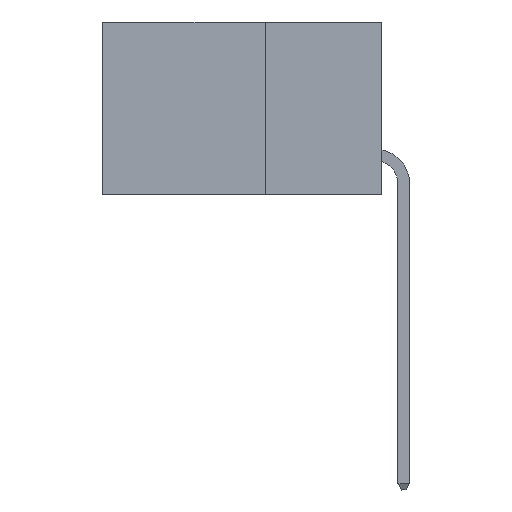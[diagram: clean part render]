
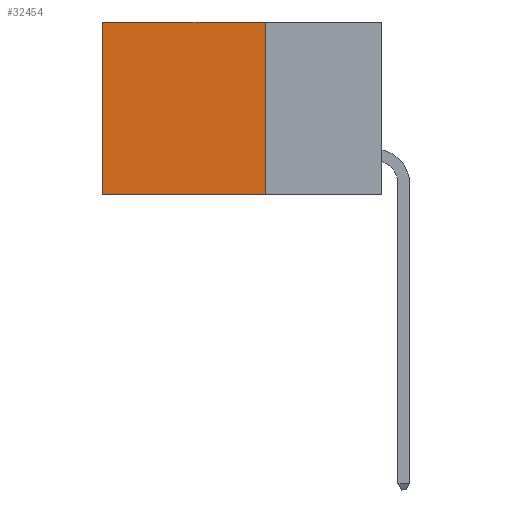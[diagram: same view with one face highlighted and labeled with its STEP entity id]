
A CAD part, left-side view. The second image highlights one B-rep face of the part: STEP entity #32454.
In plain terms, the highlighted planar face has unit normal (-1, 0, 0).
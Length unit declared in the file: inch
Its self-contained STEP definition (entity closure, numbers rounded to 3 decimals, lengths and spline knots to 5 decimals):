
#562 = CARTESIAN_POINT ( 'NONE',  ( 0.2875, 0.25, -0.37 ) ) ;
#2887 = CARTESIAN_POINT ( 'NONE',  ( 0.2875, 0.25, 0. ) ) ;
#3276 = LINE ( 'NONE', #2887, #10043 ) ;
#3632 = VECTOR ( 'NONE', #9396, 39.37008 ) ;
#3979 = CARTESIAN_POINT ( 'NONE',  ( 0.2875, 0.25, 0. ) ) ;
#5584 = VERTEX_POINT ( 'NONE', #30612 ) ;
#6220 = ORIENTED_EDGE ( 'NONE', *, *, #30101, .T. ) ;
#6611 = EDGE_LOOP ( 'NONE', ( #34724, #22418, #9302, #6220 ) ) ;
#6703 = DIRECTION ( 'NONE',  ( 1., 0., 0. ) ) ;
#8087 = DIRECTION ( 'NONE',  ( 0., 1., 0. ) ) ;
#8791 = VECTOR ( 'NONE', #34684, 39.37008 ) ;
#9302 = ORIENTED_EDGE ( 'NONE', *, *, #34766, .F. ) ;
#9396 = DIRECTION ( 'NONE',  ( 0., 0., -1. ) ) ;
#10043 = VECTOR ( 'NONE', #16266, 39.37008 ) ;
#10586 = FACE_OUTER_BOUND ( 'NONE', #6611, .T. ) ;
#15884 = CARTESIAN_POINT ( 'NONE',  ( 0.2875, 0.25, 0. ) ) ;
#15912 = LINE ( 'NONE', #15884, #8791 ) ;
#16266 = DIRECTION ( 'NONE',  ( 0., 0., -1. ) ) ;
#17108 = CARTESIAN_POINT ( 'NONE',  ( 0.2875, 0.6, 0. ) ) ;
#17117 = CARTESIAN_POINT ( 'NONE',  ( 0.2875, 0.6, 0. ) ) ;
#17743 = LINE ( 'NONE', #24245, #32455 ) ;
#17891 = VERTEX_POINT ( 'NONE', #562 ) ;
#19623 = EDGE_CURVE ( 'NONE', #17891, #21987, #17743, .T. ) ;
#19819 = DIRECTION ( 'NONE',  ( 0., 0., -1. ) ) ;
#20432 = LINE ( 'NONE', #17108, #3632 ) ;
#21987 = VERTEX_POINT ( 'NONE', #29464 ) ;
#22418 = ORIENTED_EDGE ( 'NONE', *, *, #19623, .F. ) ;
#24245 = CARTESIAN_POINT ( 'NONE',  ( 0.2875, 0.25, -0.37 ) ) ;
#24442 = AXIS2_PLACEMENT_3D ( 'NONE', #3979, #6703, #19819 ) ;
#25900 = EDGE_CURVE ( 'NONE', #28448, #21987, #20432, .T. ) ;
#27335 = PLANE ( 'NONE',  #24442 ) ;
#28448 = VERTEX_POINT ( 'NONE', #17117 ) ;
#29464 = CARTESIAN_POINT ( 'NONE',  ( 0.2875, 0.6, -0.37 ) ) ;
#30101 = EDGE_CURVE ( 'NONE', #5584, #28448, #15912, .T. ) ;
#30612 = CARTESIAN_POINT ( 'NONE',  ( 0.2875, 0.25, 0. ) ) ;
#32454 = ADVANCED_FACE ( 'NONE', ( #10586 ), #27335, .F. ) ;
#32455 = VECTOR ( 'NONE', #8087, 39.37008 ) ;
#34684 = DIRECTION ( 'NONE',  ( 0., 1., 0. ) ) ;
#34724 = ORIENTED_EDGE ( 'NONE', *, *, #25900, .T. ) ;
#34766 = EDGE_CURVE ( 'NONE', #5584, #17891, #3276, .T. ) ;
